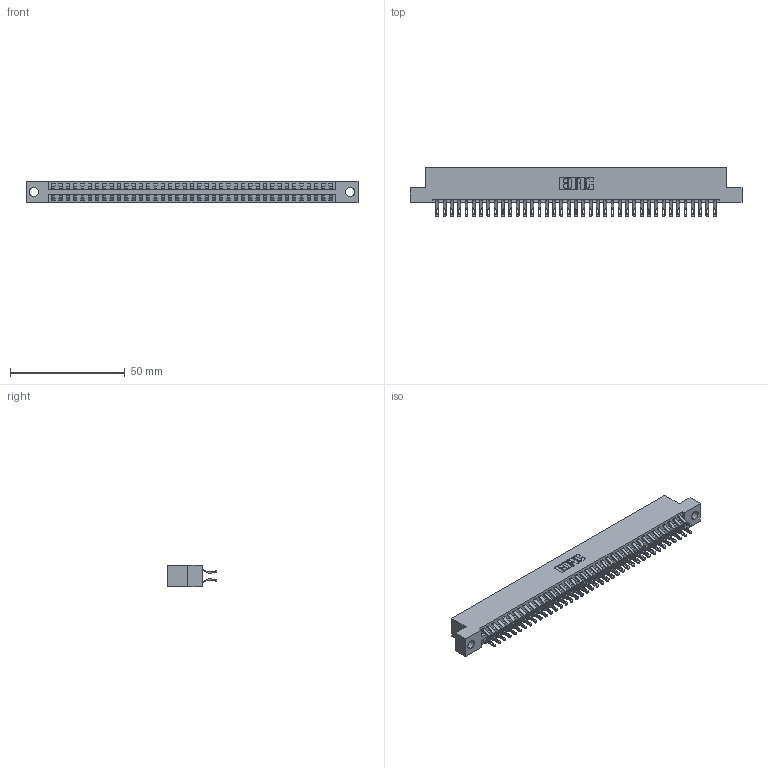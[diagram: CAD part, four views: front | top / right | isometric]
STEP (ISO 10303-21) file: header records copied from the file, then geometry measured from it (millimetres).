
FILE_DESCRIPTION (( 'STEP AP203' ), '1' );
FILE_NAME ('346-078-555-204.STEP', '2022-05-25T14:21:15', ( '' ), ( '' ), 'SwSTEP 2.0', 'SolidWorks 2020', '' );
FILE_SCHEMA (( 'CONFIG_CONTROL_DESIGN' ));
Length unit declared in the file: inch
Products named in the file (3): 346 Part_Flush Mounting Lugs - 0.156 Dia-TH; 346-078-555-204; 345-292-001_555 Tail
Assembly tree (79 placements, depth 2):
  346-078-555-204
    346 Part_Flush Mounting Lugs - 0.156 Dia-TH
    345-292-001_555 Tail  x78
Bounding box: 144.4 x 21.46 x 9.4 mm (x, y, z)
Volume: 14177.7 mm3; surface area: 20095.4 mm2
Topology: 79 solids, 79 shells, 4660 faces, 14639 edges, 9758 vertices
Faces by surface type: plane 2664, cylinder 1996
Entity records: 26601 total; most frequent: CARTESIAN_POINT 4428, ORIENTED_EDGE 4330, DIRECTION 3921, EDGE_CURVE 2165, LINE 1857, VECTOR 1857, VERTEX_POINT 1442, AXIS2_PLACEMENT_3D 1032
